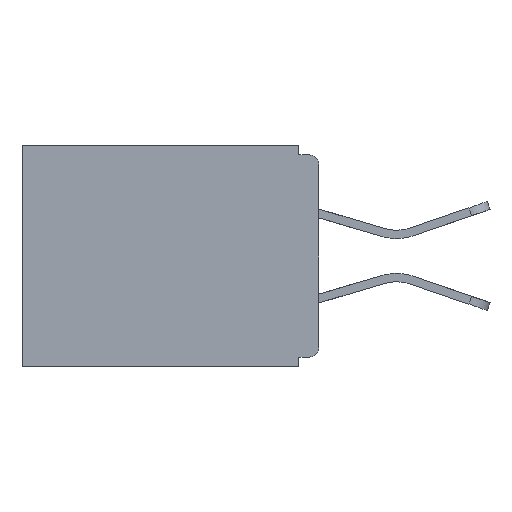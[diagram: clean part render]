
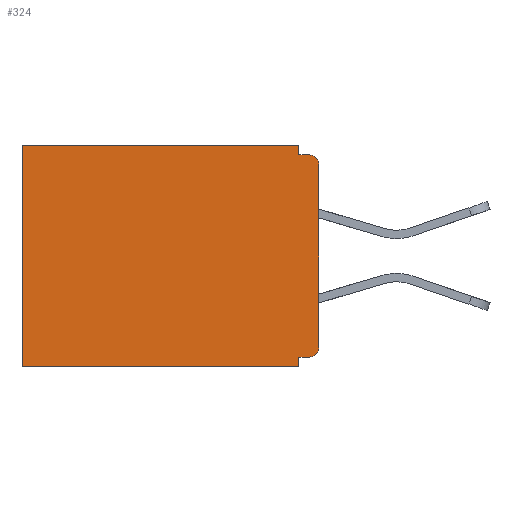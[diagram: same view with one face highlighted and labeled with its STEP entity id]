
A CAD part, left-side view. The second image highlights one B-rep face of the part: STEP entity #324.
In plain terms, the highlighted planar face has unit normal (-1, 0, 0).
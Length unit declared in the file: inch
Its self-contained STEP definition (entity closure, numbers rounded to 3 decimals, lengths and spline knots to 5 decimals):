
#92 = EDGE_CURVE ( 'NONE', #582, #13444, #16363, .T. ) ;
#116 = CARTESIAN_POINT ( 'NONE',  ( 0.298, 0.031, -0.015 ) ) ;
#238 = LINE ( 'NONE', #15211, #7161 ) ;
#324 = ADVANCED_FACE ( 'NONE', ( #8167 ), #12534, .F. ) ;
#440 = CARTESIAN_POINT ( 'NONE',  ( 0.298, 0.015, -0.03 ) ) ;
#582 = VERTEX_POINT ( 'NONE', #6189 ) ;
#627 = EDGE_CURVE ( 'NONE', #7528, #15997, #238, .T. ) ;
#922 = CARTESIAN_POINT ( 'NONE',  ( 0.298, 0., 0. ) ) ;
#1711 = DIRECTION ( 'NONE',  ( 0., 0., -1. ) ) ;
#1805 = CARTESIAN_POINT ( 'NONE',  ( 0.298, 0., -0.313 ) ) ;
#1883 = ORIENTED_EDGE ( 'NONE', *, *, #15117, .F. ) ;
#2124 = DIRECTION ( 'NONE',  ( 0., -1., 0. ) ) ;
#2146 = CIRCLE ( 'NONE', #16231, 0.015 ) ;
#2820 = AXIS2_PLACEMENT_3D ( 'NONE', #6483, #12593, #7914 ) ;
#3131 = VECTOR ( 'NONE', #14513, 39.37008 ) ;
#3442 = VERTEX_POINT ( 'NONE', #12947 ) ;
#3464 = VECTOR ( 'NONE', #11808, 39.37008 ) ;
#3918 = LINE ( 'NONE', #16087, #17872 ) ;
#4168 = ORIENTED_EDGE ( 'NONE', *, *, #13741, .T. ) ;
#4181 = ORIENTED_EDGE ( 'NONE', *, *, #627, .F. ) ;
#4242 = VERTEX_POINT ( 'NONE', #17656 ) ;
#4503 = LINE ( 'NONE', #16295, #9760 ) ;
#4567 = CARTESIAN_POINT ( 'NONE',  ( 0.298, 0.46, 0. ) ) ;
#4685 = EDGE_CURVE ( 'NONE', #5662, #7058, #5664, .T. ) ;
#4832 = EDGE_CURVE ( 'NONE', #15997, #4242, #7080, .T. ) ;
#5060 = DIRECTION ( 'NONE',  ( -1., 0., 0. ) ) ;
#5662 = VERTEX_POINT ( 'NONE', #4567 ) ;
#5664 = LINE ( 'NONE', #11028, #15302 ) ;
#6189 = CARTESIAN_POINT ( 'NONE',  ( 0.298, 0.015, -0.328 ) ) ;
#6483 = CARTESIAN_POINT ( 'NONE',  ( 0.298, 0., 0. ) ) ;
#6727 = DIRECTION ( 'NONE',  ( 0., 1., 0. ) ) ;
#7058 = VERTEX_POINT ( 'NONE', #9387 ) ;
#7080 = LINE ( 'NONE', #18987, #15998 ) ;
#7161 = VECTOR ( 'NONE', #12109, 39.37008 ) ;
#7437 = LINE ( 'NONE', #922, #3131 ) ;
#7467 = ORIENTED_EDGE ( 'NONE', *, *, #13083, .F. ) ;
#7528 = VERTEX_POINT ( 'NONE', #18845 ) ;
#7914 = DIRECTION ( 'NONE',  ( 0., 0., -1. ) ) ;
#8167 = FACE_OUTER_BOUND ( 'NONE', #18962, .T. ) ;
#8484 = LINE ( 'NONE', #16410, #3464 ) ;
#9387 = CARTESIAN_POINT ( 'NONE',  ( 0.298, 0.46, -0.343 ) ) ;
#9460 = LINE ( 'NONE', #15762, #14014 ) ;
#9760 = VECTOR ( 'NONE', #18412, 39.37008 ) ;
#10055 = ORIENTED_EDGE ( 'NONE', *, *, #17840, .T. ) ;
#10937 = DIRECTION ( 'NONE',  ( -1., 0., 0. ) ) ;
#11028 = CARTESIAN_POINT ( 'NONE',  ( 0.298, 0.46, 0. ) ) ;
#11808 = DIRECTION ( 'NONE',  ( 0., 1., 0. ) ) ;
#12109 = DIRECTION ( 'NONE',  ( 0., 0., -1. ) ) ;
#12534 = PLANE ( 'NONE',  #2820 ) ;
#12559 = DIRECTION ( 'NONE',  ( 0., 0., -1. ) ) ;
#12593 = DIRECTION ( 'NONE',  ( 1., 0., 0. ) ) ;
#12759 = EDGE_CURVE ( 'NONE', #3442, #14064, #9460, .T. ) ;
#12947 = CARTESIAN_POINT ( 'NONE',  ( 0.298, 0.031, -0.328 ) ) ;
#13083 = EDGE_CURVE ( 'NONE', #15653, #13444, #7437, .T. ) ;
#13381 = ORIENTED_EDGE ( 'NONE', *, *, #12759, .F. ) ;
#13444 = VERTEX_POINT ( 'NONE', #1805 ) ;
#13604 = CARTESIAN_POINT ( 'NONE',  ( 0.298, 0., -0.03 ) ) ;
#13741 = EDGE_CURVE ( 'NONE', #15653, #4242, #2146, .T. ) ;
#14014 = VECTOR ( 'NONE', #19328, 39.37008 ) ;
#14064 = VERTEX_POINT ( 'NONE', #14584 ) ;
#14513 = DIRECTION ( 'NONE',  ( 0., 0., -1. ) ) ;
#14584 = CARTESIAN_POINT ( 'NONE',  ( 0.298, 0.031, -0.343 ) ) ;
#15117 = EDGE_CURVE ( 'NONE', #582, #3442, #4503, .T. ) ;
#15211 = CARTESIAN_POINT ( 'NONE',  ( 0.298, 0.031, -0.343 ) ) ;
#15302 = VECTOR ( 'NONE', #12559, 39.37008 ) ;
#15622 = DIRECTION ( 'NONE',  ( 0., 0., -1. ) ) ;
#15653 = VERTEX_POINT ( 'NONE', #13604 ) ;
#15656 = CARTESIAN_POINT ( 'NONE',  ( 0.298, 0.015, -0.313 ) ) ;
#15762 = CARTESIAN_POINT ( 'NONE',  ( 0.298, 0.031, -0.343 ) ) ;
#15997 = VERTEX_POINT ( 'NONE', #116 ) ;
#15998 = VECTOR ( 'NONE', #2124, 39.37008 ) ;
#16087 = CARTESIAN_POINT ( 'NONE',  ( 0.298, 0., 0. ) ) ;
#16231 = AXIS2_PLACEMENT_3D ( 'NONE', #440, #5060, #15622 ) ;
#16295 = CARTESIAN_POINT ( 'NONE',  ( 0.298, 0., -0.328 ) ) ;
#16363 = CIRCLE ( 'NONE', #18937, 0.015 ) ;
#16410 = CARTESIAN_POINT ( 'NONE',  ( 0.298, 0., -0.343 ) ) ;
#16735 = ORIENTED_EDGE ( 'NONE', *, *, #4685, .T. ) ;
#17656 = CARTESIAN_POINT ( 'NONE',  ( 0.298, 0.015, -0.015 ) ) ;
#17840 = EDGE_CURVE ( 'NONE', #7528, #5662, #3918, .T. ) ;
#17872 = VECTOR ( 'NONE', #6727, 39.37008 ) ;
#18412 = DIRECTION ( 'NONE',  ( 0., 1., 0. ) ) ;
#18820 = ORIENTED_EDGE ( 'NONE', *, *, #92, .T. ) ;
#18845 = CARTESIAN_POINT ( 'NONE',  ( 0.298, 0.031, 0. ) ) ;
#18937 = AXIS2_PLACEMENT_3D ( 'NONE', #15656, #10937, #1711 ) ;
#18962 = EDGE_LOOP ( 'NONE', ( #4168, #19584, #4181, #10055, #16735, #19689, #13381, #1883, #18820, #7467 ) ) ;
#18987 = CARTESIAN_POINT ( 'NONE',  ( 0.298, 0., -0.015 ) ) ;
#19328 = DIRECTION ( 'NONE',  ( 0., 0., -1. ) ) ;
#19584 = ORIENTED_EDGE ( 'NONE', *, *, #4832, .F. ) ;
#19689 = ORIENTED_EDGE ( 'NONE', *, *, #19876, .F. ) ;
#19876 = EDGE_CURVE ( 'NONE', #14064, #7058, #8484, .T. ) ;
